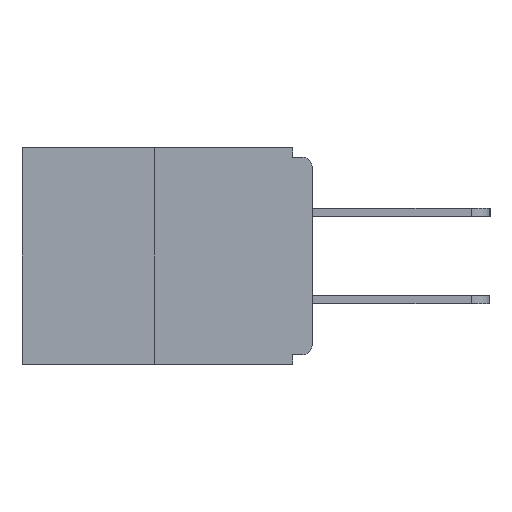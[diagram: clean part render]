
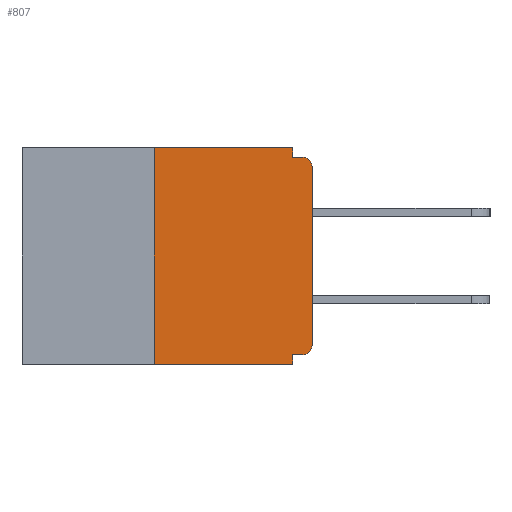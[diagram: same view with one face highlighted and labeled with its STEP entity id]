
A CAD part, left-side view. The second image highlights one B-rep face of the part: STEP entity #807.
In plain terms, the highlighted planar face has unit normal (-1, 0, 0).
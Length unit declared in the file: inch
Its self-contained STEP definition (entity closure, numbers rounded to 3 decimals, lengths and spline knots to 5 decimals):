
#23 = VECTOR ( 'NONE', #2425, 39.37008 ) ;
#292 = VECTOR ( 'NONE', #1566, 39.37008 ) ;
#571 = ORIENTED_EDGE ( 'NONE', *, *, #11436, .F. ) ;
#807 = ADVANCED_FACE ( 'NONE', ( #4959 ), #13658, .F. ) ;
#905 = VERTEX_POINT ( 'NONE', #3124 ) ;
#1143 = CARTESIAN_POINT ( 'NONE',  ( 0., 0.25, 0. ) ) ;
#1162 = CARTESIAN_POINT ( 'NONE',  ( 0., 0.015, -0.015 ) ) ;
#1286 = DIRECTION ( 'NONE',  ( 0., 0., 1. ) ) ;
#1484 = DIRECTION ( 'NONE',  ( 0., 0., -1. ) ) ;
#1522 = EDGE_CURVE ( 'NONE', #9804, #10741, #3983, .T. ) ;
#1566 = DIRECTION ( 'NONE',  ( 0., -1., 0. ) ) ;
#1612 = CARTESIAN_POINT ( 'NONE',  ( 0., 0.031, -0.343 ) ) ;
#1801 = LINE ( 'NONE', #14807, #292 ) ;
#2372 = CARTESIAN_POINT ( 'NONE',  ( 0., 0.031, 0. ) ) ;
#2425 = DIRECTION ( 'NONE',  ( 0., 0., -1. ) ) ;
#2440 = EDGE_CURVE ( 'NONE', #6441, #8833, #13703, .T. ) ;
#2449 = AXIS2_PLACEMENT_3D ( 'NONE', #6861, #6754, #4272 ) ;
#2606 = LINE ( 'NONE', #12556, #3004 ) ;
#2857 = AXIS2_PLACEMENT_3D ( 'NONE', #11417, #8781, #1484 ) ;
#2940 = EDGE_LOOP ( 'NONE', ( #4436, #6496, #8468, #571, #15035, #13755, #6662, #12332, #14210, #14689 ) ) ;
#3004 = VECTOR ( 'NONE', #5246, 39.37008 ) ;
#3124 = CARTESIAN_POINT ( 'NONE',  ( 0., 0.031, -0.328 ) ) ;
#3127 = CARTESIAN_POINT ( 'NONE',  ( 0., 0.031, -0.015 ) ) ;
#3349 = DIRECTION ( 'NONE',  ( 0., 1., 0. ) ) ;
#3657 = VERTEX_POINT ( 'NONE', #6964 ) ;
#3914 = EDGE_CURVE ( 'NONE', #4413, #905, #6930, .T. ) ;
#3983 = LINE ( 'NONE', #13365, #7608 ) ;
#4172 = CIRCLE ( 'NONE', #15516, 0.015 ) ;
#4272 = DIRECTION ( 'NONE',  ( 0., 0., -1. ) ) ;
#4413 = VERTEX_POINT ( 'NONE', #11573 ) ;
#4436 = ORIENTED_EDGE ( 'NONE', *, *, #14509, .F. ) ;
#4486 = CARTESIAN_POINT ( 'NONE',  ( 0., 0., -0.313 ) ) ;
#4959 = FACE_OUTER_BOUND ( 'NONE', #2940, .T. ) ;
#5246 = DIRECTION ( 'NONE',  ( 0., 0., -1. ) ) ;
#5424 = LINE ( 'NONE', #9263, #14023 ) ;
#6051 = DIRECTION ( 'NONE',  ( -1., 0., 0. ) ) ;
#6313 = VERTEX_POINT ( 'NONE', #4486 ) ;
#6441 = VERTEX_POINT ( 'NONE', #12565 ) ;
#6488 = EDGE_CURVE ( 'NONE', #9804, #9081, #7289, .T. ) ;
#6496 = ORIENTED_EDGE ( 'NONE', *, *, #6488, .F. ) ;
#6662 = ORIENTED_EDGE ( 'NONE', *, *, #13879, .T. ) ;
#6754 = DIRECTION ( 'NONE',  ( -1., 0., 0. ) ) ;
#6861 = CARTESIAN_POINT ( 'NONE',  ( 0., 0.015, -0.313 ) ) ;
#6930 = LINE ( 'NONE', #10619, #15543 ) ;
#6964 = CARTESIAN_POINT ( 'NONE',  ( 0., 0., -0.03 ) ) ;
#7289 = LINE ( 'NONE', #1143, #11891 ) ;
#7608 = VECTOR ( 'NONE', #12139, 39.37008 ) ;
#7978 = CARTESIAN_POINT ( 'NONE',  ( 0., 0., 0. ) ) ;
#8129 = DIRECTION ( 'NONE',  ( 0., 0., 1. ) ) ;
#8329 = EDGE_CURVE ( 'NONE', #4413, #6313, #12982, .T. ) ;
#8468 = ORIENTED_EDGE ( 'NONE', *, *, #1522, .T. ) ;
#8537 = CARTESIAN_POINT ( 'NONE',  ( 0., 0.015, -0.03 ) ) ;
#8781 = DIRECTION ( 'NONE',  ( 1., 0., 0. ) ) ;
#8833 = VERTEX_POINT ( 'NONE', #3127 ) ;
#9081 = VERTEX_POINT ( 'NONE', #11081 ) ;
#9110 = EDGE_CURVE ( 'NONE', #3657, #9338, #4172, .T. ) ;
#9263 = CARTESIAN_POINT ( 'NONE',  ( 0., 0., -0.015 ) ) ;
#9338 = VERTEX_POINT ( 'NONE', #1162 ) ;
#9363 = DIRECTION ( 'NONE',  ( 0., -1., 0. ) ) ;
#9804 = VERTEX_POINT ( 'NONE', #10792 ) ;
#10619 = CARTESIAN_POINT ( 'NONE',  ( 0., 0., -0.328 ) ) ;
#10741 = VERTEX_POINT ( 'NONE', #1612 ) ;
#10792 = CARTESIAN_POINT ( 'NONE',  ( 0., 0.25, -0.343 ) ) ;
#11081 = CARTESIAN_POINT ( 'NONE',  ( 0., 0.25, 0. ) ) ;
#11339 = VECTOR ( 'NONE', #8129, 39.37008 ) ;
#11417 = CARTESIAN_POINT ( 'NONE',  ( 0., 0.46, 0. ) ) ;
#11436 = EDGE_CURVE ( 'NONE', #905, #10741, #2606, .T. ) ;
#11573 = CARTESIAN_POINT ( 'NONE',  ( 0., 0.015, -0.328 ) ) ;
#11891 = VECTOR ( 'NONE', #1286, 39.37008 ) ;
#12139 = DIRECTION ( 'NONE',  ( 0., -1., 0. ) ) ;
#12332 = ORIENTED_EDGE ( 'NONE', *, *, #9110, .T. ) ;
#12556 = CARTESIAN_POINT ( 'NONE',  ( 0., 0.031, -0.343 ) ) ;
#12565 = CARTESIAN_POINT ( 'NONE',  ( 0., 0.031, 0. ) ) ;
#12982 = CIRCLE ( 'NONE', #2449, 0.015 ) ;
#13365 = CARTESIAN_POINT ( 'NONE',  ( 0., 0.46, -0.343 ) ) ;
#13641 = EDGE_CURVE ( 'NONE', #8833, #9338, #5424, .T. ) ;
#13658 = PLANE ( 'NONE',  #2857 ) ;
#13703 = LINE ( 'NONE', #2372, #23 ) ;
#13755 = ORIENTED_EDGE ( 'NONE', *, *, #8329, .T. ) ;
#13879 = EDGE_CURVE ( 'NONE', #6313, #3657, #15153, .T. ) ;
#14023 = VECTOR ( 'NONE', #9363, 39.37008 ) ;
#14210 = ORIENTED_EDGE ( 'NONE', *, *, #13641, .F. ) ;
#14509 = EDGE_CURVE ( 'NONE', #9081, #6441, #1801, .T. ) ;
#14607 = DIRECTION ( 'NONE',  ( 0., 0., -1. ) ) ;
#14689 = ORIENTED_EDGE ( 'NONE', *, *, #2440, .F. ) ;
#14807 = CARTESIAN_POINT ( 'NONE',  ( 0., 0.46, 0. ) ) ;
#15035 = ORIENTED_EDGE ( 'NONE', *, *, #3914, .F. ) ;
#15153 = LINE ( 'NONE', #7978, #11339 ) ;
#15516 = AXIS2_PLACEMENT_3D ( 'NONE', #8537, #6051, #14607 ) ;
#15543 = VECTOR ( 'NONE', #3349, 39.37008 ) ;
